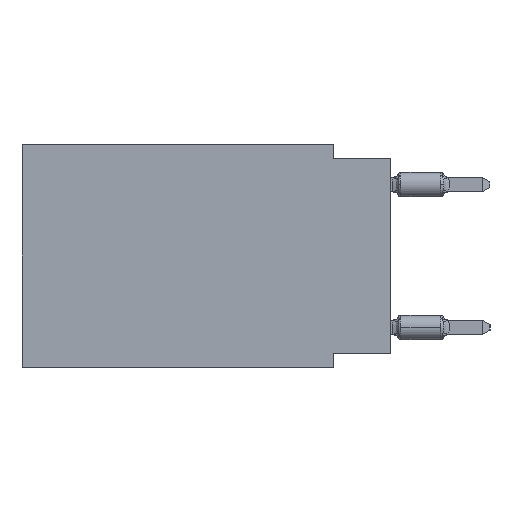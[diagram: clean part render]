
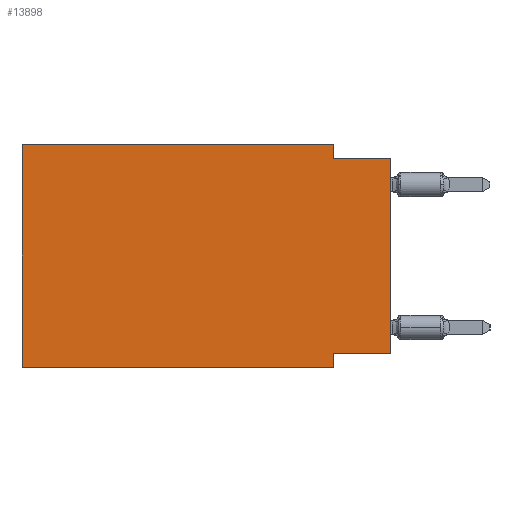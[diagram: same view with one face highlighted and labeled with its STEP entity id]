
A CAD part, left-side view. The second image highlights one B-rep face of the part: STEP entity #13898.
In plain terms, the highlighted planar face has unit normal (-1, 0, 0).
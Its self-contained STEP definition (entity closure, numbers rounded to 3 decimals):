
#440 = VECTOR ( 'NONE', #18565, 1000. ) ;
#812 = VERTEX_POINT ( 'NONE', #7077 ) ;
#856 = VERTEX_POINT ( 'NONE', #10633 ) ;
#930 = VECTOR ( 'NONE', #12018, 1000. ) ;
#1082 = LINE ( 'NONE', #6100, #21630 ) ;
#1280 = CARTESIAN_POINT ( 'NONE',  ( 0., 0., -0.635 ) ) ;
#1494 = ORIENTED_EDGE ( 'NONE', *, *, #8155, .F. ) ;
#1725 = LINE ( 'NONE', #15904, #19670 ) ;
#1874 = LINE ( 'NONE', #14212, #11932 ) ;
#2161 = EDGE_LOOP ( 'NONE', ( #5945, #12612, #5545, #15327, #12500, #21464, #8013, #1494 ) ) ;
#2537 = LINE ( 'NONE', #21616, #10721 ) ;
#3152 = DIRECTION ( 'NONE',  ( 0., 0., -1. ) ) ;
#4514 = DIRECTION ( 'NONE',  ( 0., 0., 1. ) ) ;
#5070 = CARTESIAN_POINT ( 'NONE',  ( 0., 0., -9.271 ) ) ;
#5504 = EDGE_CURVE ( 'NONE', #13457, #10128, #2537, .T. ) ;
#5545 = ORIENTED_EDGE ( 'NONE', *, *, #20988, .F. ) ;
#5945 = ORIENTED_EDGE ( 'NONE', *, *, #5504, .T. ) ;
#6073 = CARTESIAN_POINT ( 'NONE',  ( 0., 2.54, -9.271 ) ) ;
#6100 = CARTESIAN_POINT ( 'NONE',  ( 0., 16.383, 0. ) ) ;
#6728 = CARTESIAN_POINT ( 'NONE',  ( 0., 16.383, -9.906 ) ) ;
#7077 = CARTESIAN_POINT ( 'NONE',  ( 0., 2.54, 0. ) ) ;
#7440 = EDGE_CURVE ( 'NONE', #8525, #812, #1082, .T. ) ;
#7679 = VERTEX_POINT ( 'NONE', #13829 ) ;
#8013 = ORIENTED_EDGE ( 'NONE', *, *, #15612, .F. ) ;
#8048 = DIRECTION ( 'NONE',  ( 0., -1., 0. ) ) ;
#8155 = EDGE_CURVE ( 'NONE', #13457, #17601, #11973, .T. ) ;
#8525 = VERTEX_POINT ( 'NONE', #10871 ) ;
#8687 = DIRECTION ( 'NONE',  ( 0., 0., -1. ) ) ;
#9478 = DIRECTION ( 'NONE',  ( 0., 0., -1. ) ) ;
#10075 = LINE ( 'NONE', #1280, #930 ) ;
#10128 = VERTEX_POINT ( 'NONE', #18344 ) ;
#10195 = CARTESIAN_POINT ( 'NONE',  ( 0., 16.383, 0. ) ) ;
#10633 = CARTESIAN_POINT ( 'NONE',  ( 0., 2.54, -0.635 ) ) ;
#10721 = VECTOR ( 'NONE', #4514, 1000. ) ;
#10871 = CARTESIAN_POINT ( 'NONE',  ( 0., 16.383, 0. ) ) ;
#11561 = CARTESIAN_POINT ( 'NONE',  ( 0., 16.383, 0. ) ) ;
#11635 = CARTESIAN_POINT ( 'NONE',  ( 0., 0., -9.271 ) ) ;
#11688 = PLANE ( 'NONE',  #17886 ) ;
#11932 = VECTOR ( 'NONE', #17887, 1000. ) ;
#11973 = LINE ( 'NONE', #5070, #13878 ) ;
#12018 = DIRECTION ( 'NONE',  ( 0., -1., 0. ) ) ;
#12500 = ORIENTED_EDGE ( 'NONE', *, *, #19394, .F. ) ;
#12612 = ORIENTED_EDGE ( 'NONE', *, *, #12817, .F. ) ;
#12692 = CARTESIAN_POINT ( 'NONE',  ( 0., 2.54, 0. ) ) ;
#12801 = LINE ( 'NONE', #12692, #20359 ) ;
#12817 = EDGE_CURVE ( 'NONE', #856, #10128, #10075, .T. ) ;
#13457 = VERTEX_POINT ( 'NONE', #11635 ) ;
#13829 = CARTESIAN_POINT ( 'NONE',  ( 0., 2.54, -9.906 ) ) ;
#13878 = VECTOR ( 'NONE', #19196, 1000. ) ;
#13898 = ADVANCED_FACE ( 'NONE', ( #18584 ), #11688, .F. ) ;
#14212 = CARTESIAN_POINT ( 'NONE',  ( 0., 16.383, -9.906 ) ) ;
#15327 = ORIENTED_EDGE ( 'NONE', *, *, #7440, .F. ) ;
#15521 = VERTEX_POINT ( 'NONE', #6728 ) ;
#15612 = EDGE_CURVE ( 'NONE', #17601, #7679, #1725, .T. ) ;
#15904 = CARTESIAN_POINT ( 'NONE',  ( 0., 2.54, -9.906 ) ) ;
#17601 = VERTEX_POINT ( 'NONE', #6073 ) ;
#17886 = AXIS2_PLACEMENT_3D ( 'NONE', #10195, #18685, #3152 ) ;
#17887 = DIRECTION ( 'NONE',  ( 0., -1., 0. ) ) ;
#18344 = CARTESIAN_POINT ( 'NONE',  ( 0., 0., -0.635 ) ) ;
#18565 = DIRECTION ( 'NONE',  ( 0., 0., 1. ) ) ;
#18584 = FACE_OUTER_BOUND ( 'NONE', #2161, .T. ) ;
#18685 = DIRECTION ( 'NONE',  ( 1., 0., 0. ) ) ;
#19196 = DIRECTION ( 'NONE',  ( 0., 1., 0. ) ) ;
#19394 = EDGE_CURVE ( 'NONE', #15521, #8525, #20605, .T. ) ;
#19670 = VECTOR ( 'NONE', #8687, 1000. ) ;
#20359 = VECTOR ( 'NONE', #9478, 1000. ) ;
#20399 = EDGE_CURVE ( 'NONE', #15521, #7679, #1874, .T. ) ;
#20605 = LINE ( 'NONE', #11561, #440 ) ;
#20988 = EDGE_CURVE ( 'NONE', #812, #856, #12801, .T. ) ;
#21464 = ORIENTED_EDGE ( 'NONE', *, *, #20399, .T. ) ;
#21616 = CARTESIAN_POINT ( 'NONE',  ( 0., 0., 0. ) ) ;
#21630 = VECTOR ( 'NONE', #8048, 1000. ) ;
